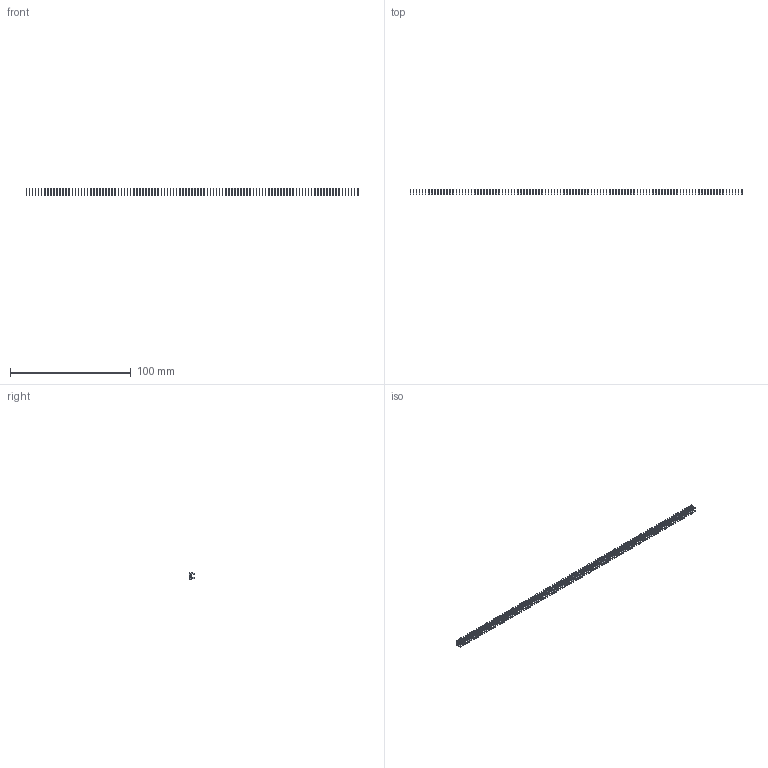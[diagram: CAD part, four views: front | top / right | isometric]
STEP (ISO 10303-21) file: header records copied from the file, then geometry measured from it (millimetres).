
FILE_DESCRIPTION (( 'STEP AP203' ), '1' );
FILE_NAME ('105-109-208-100.STEP', '2020-04-08T01:22:12', ( '' ), ( '' ), 'SwSTEP 2.0', 'SolidWorks 2016', '' );
FILE_SCHEMA (( 'CONFIG_CONTROL_DESIGN' ));
Length unit declared in the file: inch
Products named in the file (2): 105-109-208-100; 100-290-001_100-290-208
Assembly tree (109 placements, depth 2):
  105-109-208-100
    100-290-001_100-290-208  x109
Bounding box: 274.83 x 4.82 x 5.17 mm (x, y, z)
Volume: 750 mm3; surface area: 4632.1 mm2
Topology: 109 solids, 109 shells, 2725 faces, 7521 edges, 5014 vertices
Faces by surface type: plane 2398, cylinder 327
Entity records: 4445 total; most frequent: DIRECTION 349, CARTESIAN_POINT 252, CALENDAR_DATE 228, LOCAL_TIME 228, COORDINATED_UNIVERSAL_TIME_OFFSET 228, DATE_AND_TIME 228, AXIS2_PLACEMENT_3D 143, ORIENTED_EDGE 138
